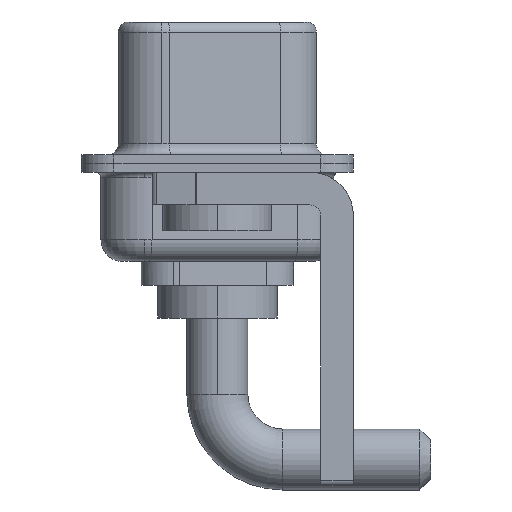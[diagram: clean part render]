
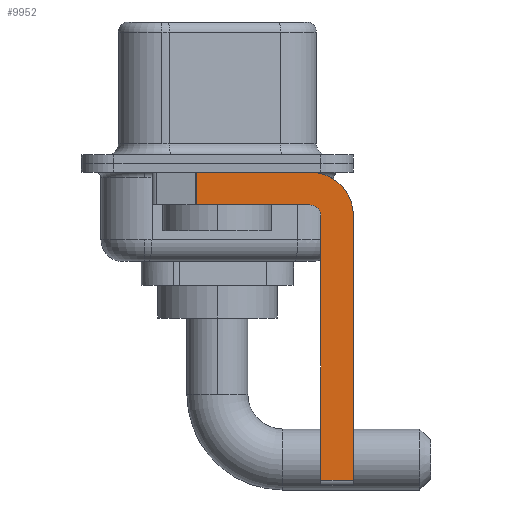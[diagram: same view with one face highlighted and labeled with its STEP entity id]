
A CAD part, left-side view. The second image highlights one B-rep face of the part: STEP entity #9952.
In plain terms, the highlighted planar face has unit normal (-1, 0, 0).
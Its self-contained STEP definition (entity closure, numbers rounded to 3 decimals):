
#130 = VECTOR ( 'NONE', #13262, 1000. ) ;
#571 = CARTESIAN_POINT ( 'NONE',  ( -2.9, -4.25, -14.55 ) ) ;
#1369 = CARTESIAN_POINT ( 'NONE',  ( -2.9, -6.25, -2.4 ) ) ;
#1531 = CARTESIAN_POINT ( 'NONE',  ( -2.9, -4.25, -1.9 ) ) ;
#1672 = EDGE_CURVE ( 'NONE', #9077, #11606, #2907, .T. ) ;
#2050 = CIRCLE ( 'NONE', #13604, 0.5 ) ;
#2394 = ORIENTED_EDGE ( 'NONE', *, *, #14191, .T. ) ;
#2490 = EDGE_CURVE ( 'NONE', #14601, #16307, #14119, .T. ) ;
#2624 = LINE ( 'NONE', #1369, #6703 ) ;
#2708 = EDGE_CURVE ( 'NONE', #12710, #6226, #2050, .T. ) ;
#2907 = LINE ( 'NONE', #6990, #130 ) ;
#2946 = DIRECTION ( 'NONE',  ( 0., 0., -1. ) ) ;
#3401 = EDGE_CURVE ( 'NONE', #6466, #12710, #9586, .T. ) ;
#4208 = PLANE ( 'NONE',  #4309 ) ;
#4309 = AXIS2_PLACEMENT_3D ( 'NONE', #9316, #7014, #2946 ) ;
#4454 = ORIENTED_EDGE ( 'NONE', *, *, #8938, .F. ) ;
#4663 = DIRECTION ( 'NONE',  ( 0., -1., 0. ) ) ;
#4750 = ORIENTED_EDGE ( 'NONE', *, *, #2490, .F. ) ;
#4761 = DIRECTION ( 'NONE',  ( 0., 0., 1. ) ) ;
#4804 = CARTESIAN_POINT ( 'NONE',  ( -2.9, -6.25, -2.4 ) ) ;
#5106 = CARTESIAN_POINT ( 'NONE',  ( -2.9, 0.978, -1.9 ) ) ;
#5240 = CARTESIAN_POINT ( 'NONE',  ( -2.9, -4.25, -0.4 ) ) ;
#5538 = DIRECTION ( 'NONE',  ( 0., 1., 0. ) ) ;
#5621 = CARTESIAN_POINT ( 'NONE',  ( -2.9, 0.978, -0.4 ) ) ;
#5902 = CARTESIAN_POINT ( 'NONE',  ( -2.9, 3., -0.4 ) ) ;
#6028 = CARTESIAN_POINT ( 'NONE',  ( -2.9, -4.75, -14.55 ) ) ;
#6226 = VERTEX_POINT ( 'NONE', #1531 ) ;
#6277 = EDGE_CURVE ( 'NONE', #6226, #11606, #10571, .T. ) ;
#6466 = VERTEX_POINT ( 'NONE', #6028 ) ;
#6703 = VECTOR ( 'NONE', #12875, 1000. ) ;
#6889 = CARTESIAN_POINT ( 'NONE',  ( -2.9, -4.75, -14.8 ) ) ;
#6990 = CARTESIAN_POINT ( 'NONE',  ( -2.9, 0.978, -1.9 ) ) ;
#7014 = DIRECTION ( 'NONE',  ( 1., 0., 0. ) ) ;
#7113 = ORIENTED_EDGE ( 'NONE', *, *, #1672, .T. ) ;
#7835 = ORIENTED_EDGE ( 'NONE', *, *, #6277, .F. ) ;
#7867 = CARTESIAN_POINT ( 'NONE',  ( -2.9, -4.25, -2.4 ) ) ;
#7869 = VERTEX_POINT ( 'NONE', #14675 ) ;
#7908 = AXIS2_PLACEMENT_3D ( 'NONE', #7867, #8746, #13904 ) ;
#8292 = ORIENTED_EDGE ( 'NONE', *, *, #2708, .F. ) ;
#8746 = DIRECTION ( 'NONE',  ( 1., 0., 0. ) ) ;
#8938 = EDGE_CURVE ( 'NONE', #16307, #7869, #2624, .T. ) ;
#9011 = VECTOR ( 'NONE', #10677, 1000. ) ;
#9077 = VERTEX_POINT ( 'NONE', #5621 ) ;
#9316 = CARTESIAN_POINT ( 'NONE',  ( -2.9, -4.25, -2.4 ) ) ;
#9586 = LINE ( 'NONE', #6889, #9011 ) ;
#9648 = ORIENTED_EDGE ( 'NONE', *, *, #3401, .F. ) ;
#9800 = VECTOR ( 'NONE', #16171, 1000. ) ;
#9952 = ADVANCED_FACE ( 'NONE', ( #15649 ), #4208, .F. ) ;
#10571 = LINE ( 'NONE', #15719, #13995 ) ;
#10677 = DIRECTION ( 'NONE',  ( 0., 0., 1. ) ) ;
#11140 = DIRECTION ( 'NONE',  ( -1., 0., 0. ) ) ;
#11606 = VERTEX_POINT ( 'NONE', #5106 ) ;
#12298 = LINE ( 'NONE', #5902, #9800 ) ;
#12443 = VECTOR ( 'NONE', #4663, 1000. ) ;
#12655 = EDGE_LOOP ( 'NONE', ( #13936, #7113, #7835, #8292, #9648, #2394, #4454, #4750 ) ) ;
#12710 = VERTEX_POINT ( 'NONE', #15774 ) ;
#12875 = DIRECTION ( 'NONE',  ( 0., 0., -1. ) ) ;
#13262 = DIRECTION ( 'NONE',  ( 0., 0., -1. ) ) ;
#13604 = AXIS2_PLACEMENT_3D ( 'NONE', #15038, #11140, #4761 ) ;
#13904 = DIRECTION ( 'NONE',  ( 0., 0., -1. ) ) ;
#13936 = ORIENTED_EDGE ( 'NONE', *, *, #16242, .F. ) ;
#13995 = VECTOR ( 'NONE', #5538, 1000. ) ;
#14119 = CIRCLE ( 'NONE', #7908, 2. ) ;
#14191 = EDGE_CURVE ( 'NONE', #6466, #7869, #16102, .T. ) ;
#14601 = VERTEX_POINT ( 'NONE', #5240 ) ;
#14675 = CARTESIAN_POINT ( 'NONE',  ( -2.9, -6.25, -14.55 ) ) ;
#15038 = CARTESIAN_POINT ( 'NONE',  ( -2.9, -4.25, -2.4 ) ) ;
#15649 = FACE_OUTER_BOUND ( 'NONE', #12655, .T. ) ;
#15719 = CARTESIAN_POINT ( 'NONE',  ( -2.9, -4.25, -1.9 ) ) ;
#15774 = CARTESIAN_POINT ( 'NONE',  ( -2.9, -4.75, -2.4 ) ) ;
#16102 = LINE ( 'NONE', #571, #12443 ) ;
#16171 = DIRECTION ( 'NONE',  ( 0., -1., 0. ) ) ;
#16242 = EDGE_CURVE ( 'NONE', #9077, #14601, #12298, .T. ) ;
#16307 = VERTEX_POINT ( 'NONE', #4804 ) ;
